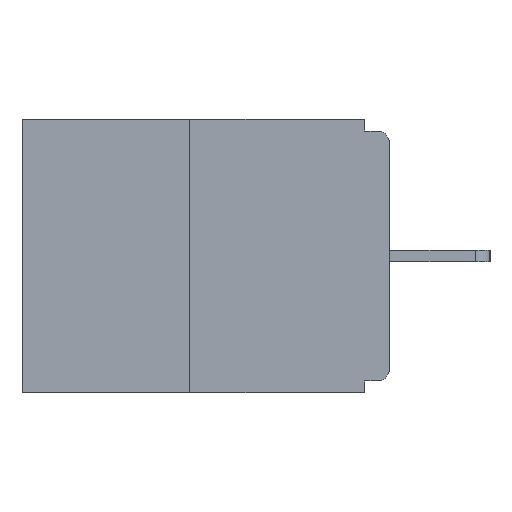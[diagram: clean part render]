
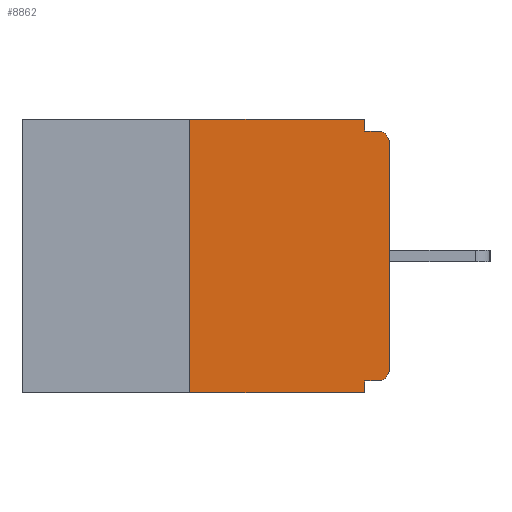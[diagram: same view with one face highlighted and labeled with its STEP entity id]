
A CAD part, left-side view. The second image highlights one B-rep face of the part: STEP entity #8862.
In plain terms, the highlighted planar face has unit normal (-1, 0, 0).
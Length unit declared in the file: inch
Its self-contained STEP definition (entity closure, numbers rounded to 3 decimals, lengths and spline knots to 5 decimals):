
#203 = VECTOR ( 'NONE', #17947, 39.37008 ) ;
#1147 = DIRECTION ( 'NONE',  ( 1., 0., 0. ) ) ;
#1495 = CARTESIAN_POINT ( 'NONE',  ( 0., 0.015, -0.313 ) ) ;
#2035 = VECTOR ( 'NONE', #21548, 39.37008 ) ;
#2094 = CARTESIAN_POINT ( 'NONE',  ( 0., 0.031, -0.343 ) ) ;
#2325 = DIRECTION ( 'NONE',  ( 0., -1., 0. ) ) ;
#2778 = ORIENTED_EDGE ( 'NONE', *, *, #21782, .T. ) ;
#3134 = LINE ( 'NONE', #3378, #203 ) ;
#3152 = PLANE ( 'NONE',  #16904 ) ;
#3194 = VERTEX_POINT ( 'NONE', #6131 ) ;
#3378 = CARTESIAN_POINT ( 'NONE',  ( 0., 0.031, 0. ) ) ;
#3654 = DIRECTION ( 'NONE',  ( 0., 0., -1. ) ) ;
#3781 = VERTEX_POINT ( 'NONE', #15843 ) ;
#3807 = EDGE_CURVE ( 'NONE', #4736, #13620, #10152, .T. ) ;
#3850 = VERTEX_POINT ( 'NONE', #21540 ) ;
#4514 = ORIENTED_EDGE ( 'NONE', *, *, #23166, .F. ) ;
#4736 = VERTEX_POINT ( 'NONE', #22710 ) ;
#6035 = ORIENTED_EDGE ( 'NONE', *, *, #13216, .T. ) ;
#6131 = CARTESIAN_POINT ( 'NONE',  ( 0., 0., -0.03 ) ) ;
#6363 = FACE_OUTER_BOUND ( 'NONE', #8049, .T. ) ;
#6611 = EDGE_CURVE ( 'NONE', #8268, #19764, #3134, .T. ) ;
#6618 = CARTESIAN_POINT ( 'NONE',  ( 0., 0., -0.015 ) ) ;
#6654 = VERTEX_POINT ( 'NONE', #6910 ) ;
#6820 = DIRECTION ( 'NONE',  ( 0., 0., 1. ) ) ;
#6910 = CARTESIAN_POINT ( 'NONE',  ( 0., 0.015, -0.015 ) ) ;
#7842 = ORIENTED_EDGE ( 'NONE', *, *, #12480, .T. ) ;
#7868 = CARTESIAN_POINT ( 'NONE',  ( 0., 0., -0.328 ) ) ;
#8049 = EDGE_LOOP ( 'NONE', ( #20374, #22296, #11200, #4514, #12775, #6035, #2778, #7842, #20423, #21868 ) ) ;
#8268 = VERTEX_POINT ( 'NONE', #8320 ) ;
#8320 = CARTESIAN_POINT ( 'NONE',  ( 0., 0.031, 0. ) ) ;
#8705 = DIRECTION ( 'NONE',  ( -1., 0., 0. ) ) ;
#8777 = DIRECTION ( 'NONE',  ( -1., 0., 0. ) ) ;
#8862 = ADVANCED_FACE ( 'NONE', ( #6363 ), #3152, .F. ) ;
#8872 = VECTOR ( 'NONE', #3654, 39.37008 ) ;
#9030 = DIRECTION ( 'NONE',  ( 0., 0., 1. ) ) ;
#9612 = EDGE_CURVE ( 'NONE', #19764, #6654, #10072, .T. ) ;
#10037 = EDGE_CURVE ( 'NONE', #4736, #3781, #20478, .T. ) ;
#10072 = LINE ( 'NONE', #6618, #23375 ) ;
#10139 = LINE ( 'NONE', #7868, #18170 ) ;
#10152 = LINE ( 'NONE', #12050, #17070 ) ;
#10378 = CARTESIAN_POINT ( 'NONE',  ( 0., 0.46, 0. ) ) ;
#11200 = ORIENTED_EDGE ( 'NONE', *, *, #10037, .T. ) ;
#11710 = CARTESIAN_POINT ( 'NONE',  ( 0., 0.015, -0.328 ) ) ;
#11794 = DIRECTION ( 'NONE',  ( 0., 1., 0. ) ) ;
#11873 = CIRCLE ( 'NONE', #21730, 0.015 ) ;
#12050 = CARTESIAN_POINT ( 'NONE',  ( 0., 0.25, 0. ) ) ;
#12480 = EDGE_CURVE ( 'NONE', #3194, #6654, #11873, .T. ) ;
#12586 = CARTESIAN_POINT ( 'NONE',  ( 0., 0.015, -0.03 ) ) ;
#12604 = LINE ( 'NONE', #20305, #17584 ) ;
#12775 = ORIENTED_EDGE ( 'NONE', *, *, #21514, .F. ) ;
#13216 = EDGE_CURVE ( 'NONE', #19287, #22777, #13803, .T. ) ;
#13620 = VERTEX_POINT ( 'NONE', #21155 ) ;
#13803 = CIRCLE ( 'NONE', #21011, 0.015 ) ;
#14294 = CARTESIAN_POINT ( 'NONE',  ( 0., 0.46, 0. ) ) ;
#14704 = CARTESIAN_POINT ( 'NONE',  ( 0., 0., -0.313 ) ) ;
#14950 = LINE ( 'NONE', #14294, #2035 ) ;
#15221 = CARTESIAN_POINT ( 'NONE',  ( 0., 0.031, -0.015 ) ) ;
#15843 = CARTESIAN_POINT ( 'NONE',  ( 0., 0.031, -0.343 ) ) ;
#15879 = DIRECTION ( 'NONE',  ( 0., -1., 0. ) ) ;
#16904 = AXIS2_PLACEMENT_3D ( 'NONE', #10378, #1147, #17633 ) ;
#17070 = VECTOR ( 'NONE', #6820, 39.37008 ) ;
#17584 = VECTOR ( 'NONE', #9030, 39.37008 ) ;
#17633 = DIRECTION ( 'NONE',  ( 0., 0., -1. ) ) ;
#17710 = DIRECTION ( 'NONE',  ( 0., 0., -1. ) ) ;
#17947 = DIRECTION ( 'NONE',  ( 0., 0., -1. ) ) ;
#18098 = VECTOR ( 'NONE', #2325, 39.37008 ) ;
#18170 = VECTOR ( 'NONE', #11794, 39.37008 ) ;
#18338 = LINE ( 'NONE', #2094, #8872 ) ;
#18578 = CARTESIAN_POINT ( 'NONE',  ( 0., 0.46, -0.343 ) ) ;
#19287 = VERTEX_POINT ( 'NONE', #11710 ) ;
#19764 = VERTEX_POINT ( 'NONE', #15221 ) ;
#20305 = CARTESIAN_POINT ( 'NONE',  ( 0., 0., 0. ) ) ;
#20374 = ORIENTED_EDGE ( 'NONE', *, *, #22357, .F. ) ;
#20423 = ORIENTED_EDGE ( 'NONE', *, *, #9612, .F. ) ;
#20478 = LINE ( 'NONE', #18578, #18098 ) ;
#20832 = DIRECTION ( 'NONE',  ( 0., 0., -1. ) ) ;
#21011 = AXIS2_PLACEMENT_3D ( 'NONE', #1495, #8705, #20832 ) ;
#21155 = CARTESIAN_POINT ( 'NONE',  ( 0., 0.25, 0. ) ) ;
#21514 = EDGE_CURVE ( 'NONE', #19287, #3850, #10139, .T. ) ;
#21540 = CARTESIAN_POINT ( 'NONE',  ( 0., 0.031, -0.328 ) ) ;
#21548 = DIRECTION ( 'NONE',  ( 0., -1., 0. ) ) ;
#21730 = AXIS2_PLACEMENT_3D ( 'NONE', #12586, #8777, #17710 ) ;
#21782 = EDGE_CURVE ( 'NONE', #22777, #3194, #12604, .T. ) ;
#21868 = ORIENTED_EDGE ( 'NONE', *, *, #6611, .F. ) ;
#22296 = ORIENTED_EDGE ( 'NONE', *, *, #3807, .F. ) ;
#22357 = EDGE_CURVE ( 'NONE', #13620, #8268, #14950, .T. ) ;
#22710 = CARTESIAN_POINT ( 'NONE',  ( 0., 0.25, -0.343 ) ) ;
#22777 = VERTEX_POINT ( 'NONE', #14704 ) ;
#23166 = EDGE_CURVE ( 'NONE', #3850, #3781, #18338, .T. ) ;
#23375 = VECTOR ( 'NONE', #15879, 39.37008 ) ;
